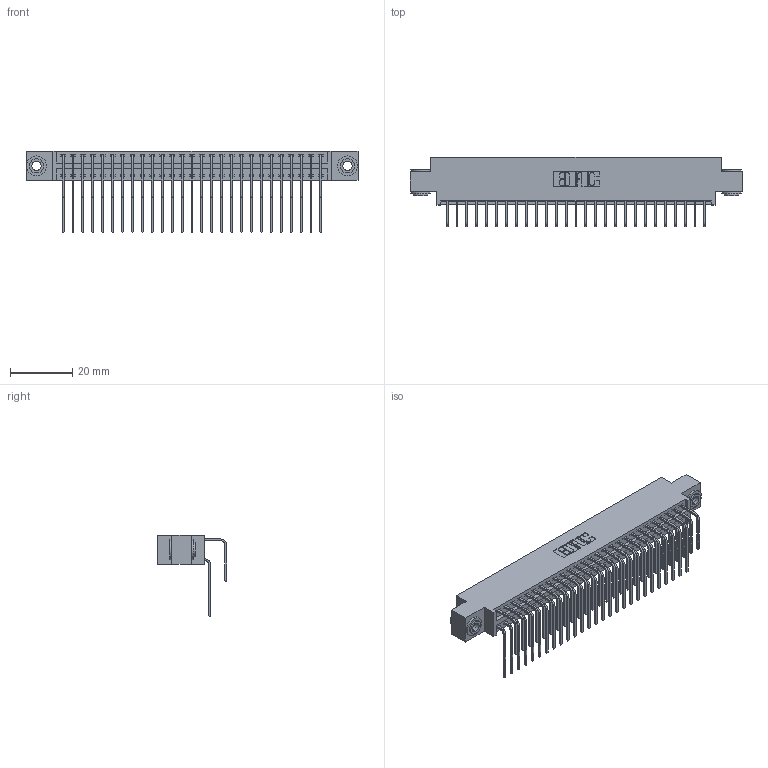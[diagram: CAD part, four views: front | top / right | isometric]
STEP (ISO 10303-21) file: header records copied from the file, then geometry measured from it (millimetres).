
FILE_DESCRIPTION (( 'STEP AP203' ), '1' );
FILE_NAME ('346-054-558-803.STEP', '2018-08-28T01:47:47', ( '' ), ( '' ), 'SwSTEP 2.0', 'SolidWorks 2016', '' );
FILE_SCHEMA (( 'CONFIG_CONTROL_DESIGN' ));
Length unit declared in the file: inch
Products named in the file (5): 345-292-001_558 559 Tail - 1; 345-292-001_558 Tail - 2; 345-250-002_345-250-002-102; 346-054-558-803; 346 Part_0.170 Offset - 0.156 Dia-TH
Assembly tree (57 placements, depth 2):
  346-054-558-803
    346 Part_0.170 Offset - 0.156 Dia-TH
    345-292-001_558 559 Tail - 1  x27
    345-292-001_558 Tail - 2  x27
    345-250-002_345-250-002-102  x2
Bounding box: 106.3 x 22.16 x 26.16 mm (x, y, z)
Volume: 10425.3 mm3; surface area: 15982.7 mm2
Topology: 57 solids, 57 shells, 3080 faces, 9111 edges, 5998 vertices
Faces by surface type: plane 2088, cylinder 984, cone 8
Entity records: 22206 total; most frequent: CARTESIAN_POINT 3710, ORIENTED_EDGE 3586, DIRECTION 3323, EDGE_CURVE 1793, VECTOR 1489, LINE 1489, VERTEX_POINT 1190, AXIS2_PLACEMENT_3D 917
